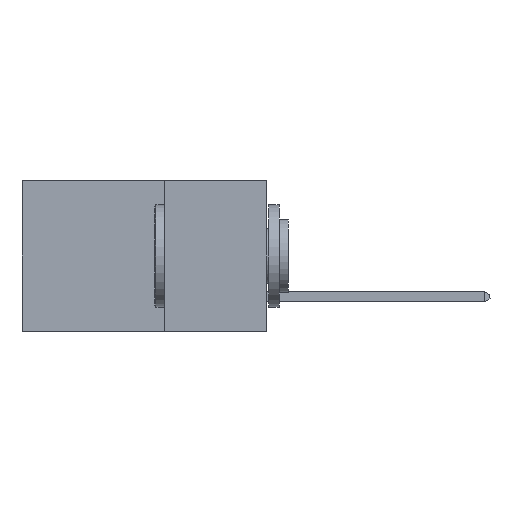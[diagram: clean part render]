
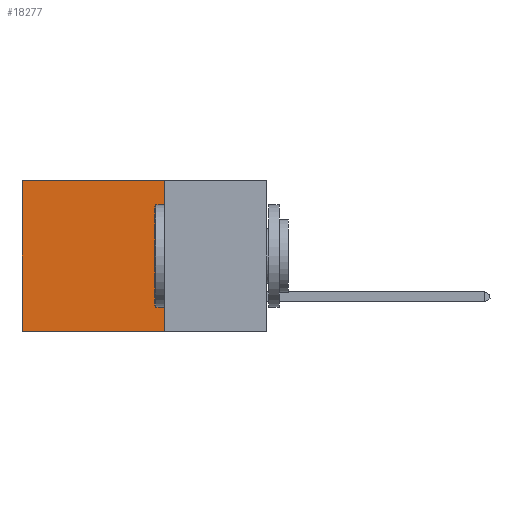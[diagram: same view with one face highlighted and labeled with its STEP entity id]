
A CAD part, left-side view. The second image highlights one B-rep face of the part: STEP entity #18277.
In plain terms, the highlighted planar face has unit normal (-1, 0, 0).
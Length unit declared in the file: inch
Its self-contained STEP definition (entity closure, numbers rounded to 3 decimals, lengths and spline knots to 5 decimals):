
#2738 = VERTEX_POINT ( 'NONE', #4184 ) ;
#2858 = CARTESIAN_POINT ( 'NONE',  ( 0.2875, 0.25, 0. ) ) ;
#4094 = LINE ( 'NONE', #28277, #8788 ) ;
#4184 = CARTESIAN_POINT ( 'NONE',  ( 0.2875, 0.25, 0. ) ) ;
#4984 = ORIENTED_EDGE ( 'NONE', *, *, #8163, .F. ) ;
#5170 = DIRECTION ( 'NONE',  ( 0., 1., 0. ) ) ;
#5727 = VERTEX_POINT ( 'NONE', #24341 ) ;
#5814 = DIRECTION ( 'NONE',  ( 0., 0., -1. ) ) ;
#6373 = PLANE ( 'NONE',  #22665 ) ;
#8163 = EDGE_CURVE ( 'NONE', #2738, #5727, #27394, .T. ) ;
#8185 = VERTEX_POINT ( 'NONE', #16441 ) ;
#8788 = VECTOR ( 'NONE', #5814, 39.37008 ) ;
#8848 = EDGE_CURVE ( 'NONE', #2738, #8185, #21112, .T. ) ;
#9786 = FACE_OUTER_BOUND ( 'NONE', #16091, .T. ) ;
#11574 = LINE ( 'NONE', #12821, #23361 ) ;
#12821 = CARTESIAN_POINT ( 'NONE',  ( 0.2875, 0.25, -0.37 ) ) ;
#13295 = DIRECTION ( 'NONE',  ( 1., 0., 0. ) ) ;
#14681 = ORIENTED_EDGE ( 'NONE', *, *, #27620, .F. ) ;
#16091 = EDGE_LOOP ( 'NONE', ( #17461, #14681, #4984, #24846 ) ) ;
#16441 = CARTESIAN_POINT ( 'NONE',  ( 0.2875, 0.6, 0. ) ) ;
#17461 = ORIENTED_EDGE ( 'NONE', *, *, #25595, .T. ) ;
#18277 = ADVANCED_FACE ( 'NONE', ( #9786 ), #6373, .F. ) ;
#18521 = CARTESIAN_POINT ( 'NONE',  ( 0.2875, 0.6, -0.37 ) ) ;
#20785 = CARTESIAN_POINT ( 'NONE',  ( 0.2875, 0.25, 0. ) ) ;
#20794 = VECTOR ( 'NONE', #27488, 39.37008 ) ;
#21112 = LINE ( 'NONE', #2858, #26285 ) ;
#22665 = AXIS2_PLACEMENT_3D ( 'NONE', #26568, #13295, #28818 ) ;
#23361 = VECTOR ( 'NONE', #28332, 39.37008 ) ;
#24341 = CARTESIAN_POINT ( 'NONE',  ( 0.2875, 0.25, -0.37 ) ) ;
#24846 = ORIENTED_EDGE ( 'NONE', *, *, #8848, .T. ) ;
#25595 = EDGE_CURVE ( 'NONE', #8185, #25883, #4094, .T. ) ;
#25883 = VERTEX_POINT ( 'NONE', #18521 ) ;
#26285 = VECTOR ( 'NONE', #5170, 39.37008 ) ;
#26568 = CARTESIAN_POINT ( 'NONE',  ( 0.2875, 0.25, 0. ) ) ;
#27394 = LINE ( 'NONE', #20785, #20794 ) ;
#27488 = DIRECTION ( 'NONE',  ( 0., 0., -1. ) ) ;
#27620 = EDGE_CURVE ( 'NONE', #5727, #25883, #11574, .T. ) ;
#28277 = CARTESIAN_POINT ( 'NONE',  ( 0.2875, 0.6, 0. ) ) ;
#28332 = DIRECTION ( 'NONE',  ( 0., 1., 0. ) ) ;
#28818 = DIRECTION ( 'NONE',  ( 0., 0., -1. ) ) ;
